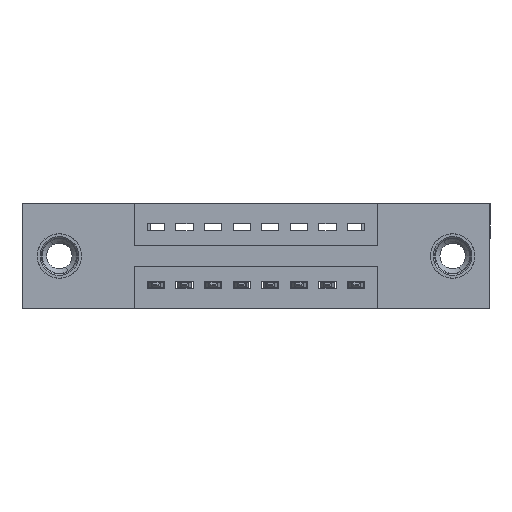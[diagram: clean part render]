
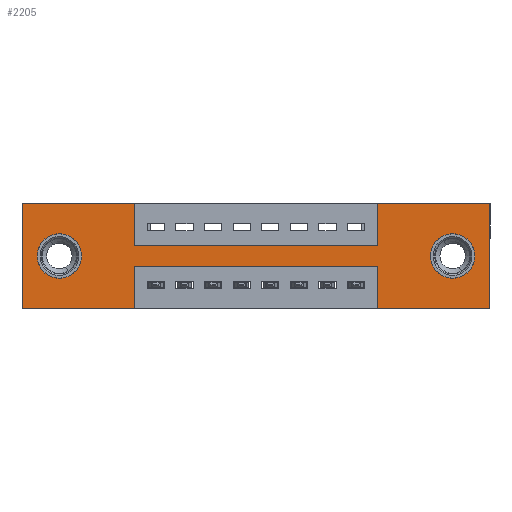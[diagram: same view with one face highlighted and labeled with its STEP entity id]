
A CAD part, front view. The second image highlights one B-rep face of the part: STEP entity #2205.
In plain terms, the highlighted planar face has unit normal (0, -1, 0).
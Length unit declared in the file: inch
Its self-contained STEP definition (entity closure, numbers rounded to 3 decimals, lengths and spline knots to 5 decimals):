
#39 = LINE ( 'NONE', #4211, #14453 ) ;
#62 = CARTESIAN_POINT ( 'NONE',  ( 1.2425, 0., -0.22 ) ) ;
#91 = DIRECTION ( 'NONE',  ( 0., 0., -1. ) ) ;
#249 = EDGE_CURVE ( 'NONE', #9400, #1229, #39, .T. ) ;
#347 = DIRECTION ( 'NONE',  ( 0., -1., 0. ) ) ;
#451 = VERTEX_POINT ( 'NONE', #10594 ) ;
#647 = DIRECTION ( 'NONE',  ( 1., 0., 0. ) ) ;
#835 = ORIENTED_EDGE ( 'NONE', *, *, #4378, .F. ) ;
#935 = CARTESIAN_POINT ( 'NONE',  ( 0.3925, 0., -0.15 ) ) ;
#944 = CARTESIAN_POINT ( 'NONE',  ( 0.3925, 0., -0.15 ) ) ;
#952 = DIRECTION ( 'NONE',  ( 0., 0., 1. ) ) ;
#1071 = ORIENTED_EDGE ( 'NONE', *, *, #7028, .F. ) ;
#1137 = EDGE_CURVE ( 'NONE', #8298, #8578, #14624, .T. ) ;
#1229 = VERTEX_POINT ( 'NONE', #12978 ) ;
#1741 = LINE ( 'NONE', #944, #14106 ) ;
#1898 = VERTEX_POINT ( 'NONE', #10661 ) ;
#2128 = VECTOR ( 'NONE', #91, 39.37008 ) ;
#2205 = ADVANCED_FACE ( 'NONE', ( #7956, #2723, #11919 ), #4549, .T. ) ;
#2332 = CARTESIAN_POINT ( 'NONE',  ( 0.3925, 0., -0.22 ) ) ;
#2347 = CARTESIAN_POINT ( 'NONE',  ( 0.3925, 0., -0.22 ) ) ;
#2353 = LINE ( 'NONE', #11452, #14713 ) ;
#2381 = DIRECTION ( 'NONE',  ( -1., 0., 0. ) ) ;
#2399 = LINE ( 'NONE', #10303, #4799 ) ;
#2546 = VERTEX_POINT ( 'NONE', #12537 ) ;
#2723 = FACE_BOUND ( 'NONE', #9117, .T. ) ;
#2801 = CARTESIAN_POINT ( 'NONE',  ( 1.2425, 0., -0.37 ) ) ;
#2914 = VECTOR ( 'NONE', #8953, 39.37008 ) ;
#2965 = CARTESIAN_POINT ( 'NONE',  ( 0.13, 0., -0.107 ) ) ;
#3148 = CARTESIAN_POINT ( 'NONE',  ( 1.2425, 0., -0.15 ) ) ;
#3235 = LINE ( 'NONE', #2801, #7509 ) ;
#3283 = DIRECTION ( 'NONE',  ( 0., 0., -1. ) ) ;
#3406 = EDGE_CURVE ( 'NONE', #14270, #4384, #13571, .T. ) ;
#3586 = CARTESIAN_POINT ( 'NONE',  ( 1.505, 0., -0.185 ) ) ;
#4086 = ORIENTED_EDGE ( 'NONE', *, *, #6741, .F. ) ;
#4158 = ORIENTED_EDGE ( 'NONE', *, *, #1137, .T. ) ;
#4211 = CARTESIAN_POINT ( 'NONE',  ( 0.3925, 0., -0.37 ) ) ;
#4248 = DIRECTION ( 'NONE',  ( 0., 1., 0. ) ) ;
#4301 = ORIENTED_EDGE ( 'NONE', *, *, #8777, .F. ) ;
#4324 = EDGE_LOOP ( 'NONE', ( #10273, #10194 ) ) ;
#4325 = CARTESIAN_POINT ( 'NONE',  ( 1.2425, 0., 0. ) ) ;
#4378 = EDGE_CURVE ( 'NONE', #1898, #5422, #9237, .T. ) ;
#4384 = VERTEX_POINT ( 'NONE', #935 ) ;
#4549 = PLANE ( 'NONE',  #11904 ) ;
#4570 = ORIENTED_EDGE ( 'NONE', *, *, #12753, .F. ) ;
#4576 = DIRECTION ( 'NONE',  ( 1., 0., 0. ) ) ;
#4799 = VECTOR ( 'NONE', #6304, 39.37008 ) ;
#4992 = ORIENTED_EDGE ( 'NONE', *, *, #15253, .F. ) ;
#5177 = DIRECTION ( 'NONE',  ( 0., 0., -1. ) ) ;
#5217 = EDGE_CURVE ( 'NONE', #8578, #8298, #11262, .T. ) ;
#5294 = VECTOR ( 'NONE', #12900, 39.37008 ) ;
#5422 = VERTEX_POINT ( 'NONE', #12130 ) ;
#5455 = ORIENTED_EDGE ( 'NONE', *, *, #3406, .F. ) ;
#5565 = AXIS2_PLACEMENT_3D ( 'NONE', #15329, #15272, #952 ) ;
#5617 = EDGE_LOOP ( 'NONE', ( #9657, #9551, #4992, #6176, #835, #10460, #4570, #8983, #5455, #1071, #4301, #4086 ) ) ;
#5782 = VECTOR ( 'NONE', #7720, 39.37008 ) ;
#6071 = CARTESIAN_POINT ( 'NONE',  ( 0.3925, 0., 0. ) ) ;
#6142 = LINE ( 'NONE', #10167, #5782 ) ;
#6176 = ORIENTED_EDGE ( 'NONE', *, *, #6725, .F. ) ;
#6304 = DIRECTION ( 'NONE',  ( 1., 0., 0. ) ) ;
#6421 = VERTEX_POINT ( 'NONE', #7242 ) ;
#6703 = VERTEX_POINT ( 'NONE', #3148 ) ;
#6725 = EDGE_CURVE ( 'NONE', #5422, #15285, #7062, .T. ) ;
#6734 = CARTESIAN_POINT ( 'NONE',  ( 0., 0., -0.37 ) ) ;
#6741 = EDGE_CURVE ( 'NONE', #1229, #10064, #6142, .T. ) ;
#6760 = CARTESIAN_POINT ( 'NONE',  ( 0., 0., 0. ) ) ;
#6899 = EDGE_CURVE ( 'NONE', #451, #2546, #13300, .T. ) ;
#7028 = EDGE_CURVE ( 'NONE', #6421, #14270, #2399, .T. ) ;
#7062 = LINE ( 'NONE', #6734, #13675 ) ;
#7128 = AXIS2_PLACEMENT_3D ( 'NONE', #7694, #4248, #12665 ) ;
#7242 = CARTESIAN_POINT ( 'NONE',  ( 0., 0., 0. ) ) ;
#7509 = VECTOR ( 'NONE', #10019, 39.37008 ) ;
#7694 = CARTESIAN_POINT ( 'NONE',  ( 0.13, 0., -0.185 ) ) ;
#7720 = DIRECTION ( 'NONE',  ( -1., 0., 0. ) ) ;
#7956 = FACE_BOUND ( 'NONE', #4324, .T. ) ;
#7976 = LINE ( 'NONE', #2332, #13248 ) ;
#8153 = AXIS2_PLACEMENT_3D ( 'NONE', #3586, #13104, #11999 ) ;
#8246 = CARTESIAN_POINT ( 'NONE',  ( 0., 0., -0.37 ) ) ;
#8298 = VERTEX_POINT ( 'NONE', #13602 ) ;
#8365 = CARTESIAN_POINT ( 'NONE',  ( 0., 0., -0.37 ) ) ;
#8460 = EDGE_CURVE ( 'NONE', #8477, #1898, #2353, .T. ) ;
#8477 = VERTEX_POINT ( 'NONE', #10200 ) ;
#8503 = LINE ( 'NONE', #6760, #2914 ) ;
#8578 = VERTEX_POINT ( 'NONE', #2965 ) ;
#8777 = EDGE_CURVE ( 'NONE', #10064, #6421, #8503, .T. ) ;
#8953 = DIRECTION ( 'NONE',  ( 0., 0., 1. ) ) ;
#8983 = ORIENTED_EDGE ( 'NONE', *, *, #10653, .F. ) ;
#8999 = ORIENTED_EDGE ( 'NONE', *, *, #5217, .T. ) ;
#9080 = DIRECTION ( 'NONE',  ( 0., 0., 1. ) ) ;
#9117 = EDGE_LOOP ( 'NONE', ( #8999, #4158 ) ) ;
#9237 = LINE ( 'NONE', #15233, #5294 ) ;
#9333 = VERTEX_POINT ( 'NONE', #62 ) ;
#9400 = VERTEX_POINT ( 'NONE', #2347 ) ;
#9522 = LINE ( 'NONE', #4325, #14956 ) ;
#9551 = ORIENTED_EDGE ( 'NONE', *, *, #13680, .F. ) ;
#9657 = ORIENTED_EDGE ( 'NONE', *, *, #249, .F. ) ;
#9946 = EDGE_CURVE ( 'NONE', #2546, #451, #14301, .T. ) ;
#10019 = DIRECTION ( 'NONE',  ( 0., 0., 1. ) ) ;
#10064 = VERTEX_POINT ( 'NONE', #8246 ) ;
#10167 = CARTESIAN_POINT ( 'NONE',  ( 0., 0., -0.37 ) ) ;
#10194 = ORIENTED_EDGE ( 'NONE', *, *, #9946, .T. ) ;
#10200 = CARTESIAN_POINT ( 'NONE',  ( 1.2425, 0., 0. ) ) ;
#10273 = ORIENTED_EDGE ( 'NONE', *, *, #6899, .T. ) ;
#10303 = CARTESIAN_POINT ( 'NONE',  ( 0., 0., 0. ) ) ;
#10460 = ORIENTED_EDGE ( 'NONE', *, *, #8460, .F. ) ;
#10594 = CARTESIAN_POINT ( 'NONE',  ( 1.505, 0., -0.107 ) ) ;
#10653 = EDGE_CURVE ( 'NONE', #4384, #6703, #1741, .T. ) ;
#10661 = CARTESIAN_POINT ( 'NONE',  ( 1.635, 0., 0. ) ) ;
#10742 = CARTESIAN_POINT ( 'NONE',  ( 0.3925, 0., 0. ) ) ;
#11262 = CIRCLE ( 'NONE', #5565, 0.078 ) ;
#11273 = CARTESIAN_POINT ( 'NONE',  ( 1.2425, 0., -0.37 ) ) ;
#11452 = CARTESIAN_POINT ( 'NONE',  ( 0., 0., 0. ) ) ;
#11904 = AXIS2_PLACEMENT_3D ( 'NONE', #8365, #347, #5177 ) ;
#11919 = FACE_OUTER_BOUND ( 'NONE', #5617, .T. ) ;
#11950 = DIRECTION ( 'NONE',  ( 0., 0., -1. ) ) ;
#11999 = DIRECTION ( 'NONE',  ( 0., 0., -1. ) ) ;
#12130 = CARTESIAN_POINT ( 'NONE',  ( 1.635, 0., -0.37 ) ) ;
#12303 = CARTESIAN_POINT ( 'NONE',  ( 1.505, 0., -0.185 ) ) ;
#12537 = CARTESIAN_POINT ( 'NONE',  ( 1.505, 0., -0.263 ) ) ;
#12665 = DIRECTION ( 'NONE',  ( 0., 0., 1. ) ) ;
#12753 = EDGE_CURVE ( 'NONE', #6703, #8477, #9522, .T. ) ;
#12900 = DIRECTION ( 'NONE',  ( 0., 0., -1. ) ) ;
#12978 = CARTESIAN_POINT ( 'NONE',  ( 0.3925, 0., -0.37 ) ) ;
#13104 = DIRECTION ( 'NONE',  ( 0., 1., 0. ) ) ;
#13248 = VECTOR ( 'NONE', #2381, 39.37008 ) ;
#13300 = CIRCLE ( 'NONE', #8153, 0.078 ) ;
#13571 = LINE ( 'NONE', #10742, #2128 ) ;
#13602 = CARTESIAN_POINT ( 'NONE',  ( 0.13, 0., -0.263 ) ) ;
#13675 = VECTOR ( 'NONE', #15062, 39.37008 ) ;
#13680 = EDGE_CURVE ( 'NONE', #9333, #9400, #7976, .T. ) ;
#14106 = VECTOR ( 'NONE', #4576, 39.37008 ) ;
#14255 = DIRECTION ( 'NONE',  ( 0., 1., 0. ) ) ;
#14270 = VERTEX_POINT ( 'NONE', #6071 ) ;
#14301 = CIRCLE ( 'NONE', #15314, 0.078 ) ;
#14453 = VECTOR ( 'NONE', #3283, 39.37008 ) ;
#14624 = CIRCLE ( 'NONE', #7128, 0.078 ) ;
#14713 = VECTOR ( 'NONE', #647, 39.37008 ) ;
#14956 = VECTOR ( 'NONE', #9080, 39.37008 ) ;
#15062 = DIRECTION ( 'NONE',  ( -1., 0., 0. ) ) ;
#15233 = CARTESIAN_POINT ( 'NONE',  ( 1.635, 0., 0. ) ) ;
#15253 = EDGE_CURVE ( 'NONE', #15285, #9333, #3235, .T. ) ;
#15272 = DIRECTION ( 'NONE',  ( 0., 1., 0. ) ) ;
#15285 = VERTEX_POINT ( 'NONE', #11273 ) ;
#15314 = AXIS2_PLACEMENT_3D ( 'NONE', #12303, #14255, #11950 ) ;
#15329 = CARTESIAN_POINT ( 'NONE',  ( 0.13, 0., -0.185 ) ) ;
